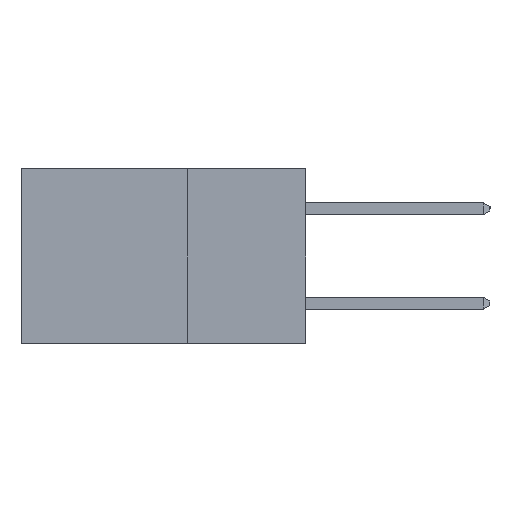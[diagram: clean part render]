
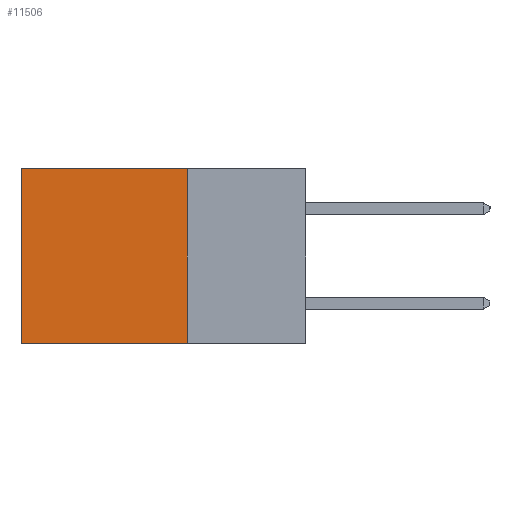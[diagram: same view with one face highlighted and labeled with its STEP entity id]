
A CAD part, left-side view. The second image highlights one B-rep face of the part: STEP entity #11506.
In plain terms, the highlighted planar face has unit normal (-1, 0, 0).
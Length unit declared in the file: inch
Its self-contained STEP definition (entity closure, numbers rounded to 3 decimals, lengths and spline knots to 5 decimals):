
#548 = VECTOR ( 'NONE', #12757, 39.37008 ) ;
#884 = ORIENTED_EDGE ( 'NONE', *, *, #16529, .T. ) ;
#2246 = CARTESIAN_POINT ( 'NONE',  ( 0.2615, 0.25, -0.37 ) ) ;
#3835 = LINE ( 'NONE', #18355, #8710 ) ;
#4700 = DIRECTION ( 'NONE',  ( 1., 0., 0. ) ) ;
#5095 = PLANE ( 'NONE',  #11170 ) ;
#5743 = ORIENTED_EDGE ( 'NONE', *, *, #10610, .F. ) ;
#5829 = LINE ( 'NONE', #16227, #17690 ) ;
#7316 = CARTESIAN_POINT ( 'NONE',  ( 0.2615, 0.6, 0. ) ) ;
#7405 = ORIENTED_EDGE ( 'NONE', *, *, #15174, .T. ) ;
#7695 = DIRECTION ( 'NONE',  ( 0., 1., 0. ) ) ;
#7808 = DIRECTION ( 'NONE',  ( 0., 1., 0. ) ) ;
#8710 = VECTOR ( 'NONE', #9820, 39.37008 ) ;
#8884 = ORIENTED_EDGE ( 'NONE', *, *, #15181, .F. ) ;
#9820 = DIRECTION ( 'NONE',  ( 0., 0., -1. ) ) ;
#10110 = VERTEX_POINT ( 'NONE', #13282 ) ;
#10532 = VERTEX_POINT ( 'NONE', #11553 ) ;
#10610 = EDGE_CURVE ( 'NONE', #14401, #10532, #5829, .T. ) ;
#10849 = LINE ( 'NONE', #15454, #18750 ) ;
#10894 = DIRECTION ( 'NONE',  ( 0., 0., -1. ) ) ;
#11170 = AXIS2_PLACEMENT_3D ( 'NONE', #13619, #4700, #10894 ) ;
#11506 = ADVANCED_FACE ( 'NONE', ( #16667 ), #5095, .F. ) ;
#11553 = CARTESIAN_POINT ( 'NONE',  ( 0.2615, 0.6, -0.37 ) ) ;
#12578 = LINE ( 'NONE', #15428, #548 ) ;
#12757 = DIRECTION ( 'NONE',  ( 0., 0., -1. ) ) ;
#13282 = CARTESIAN_POINT ( 'NONE',  ( 0.2615, 0.25, 0. ) ) ;
#13619 = CARTESIAN_POINT ( 'NONE',  ( 0.2615, 0.25, -0.37 ) ) ;
#13737 = VERTEX_POINT ( 'NONE', #7316 ) ;
#14401 = VERTEX_POINT ( 'NONE', #2246 ) ;
#15174 = EDGE_CURVE ( 'NONE', #13737, #10532, #12578, .T. ) ;
#15181 = EDGE_CURVE ( 'NONE', #10110, #14401, #3835, .T. ) ;
#15428 = CARTESIAN_POINT ( 'NONE',  ( 0.2615, 0.6, -0.37 ) ) ;
#15454 = CARTESIAN_POINT ( 'NONE',  ( 0.2615, 0.25, 0. ) ) ;
#16227 = CARTESIAN_POINT ( 'NONE',  ( 0.2615, 0.25, -0.37 ) ) ;
#16529 = EDGE_CURVE ( 'NONE', #10110, #13737, #10849, .T. ) ;
#16667 = FACE_OUTER_BOUND ( 'NONE', #18345, .T. ) ;
#17690 = VECTOR ( 'NONE', #7695, 39.37008 ) ;
#18345 = EDGE_LOOP ( 'NONE', ( #7405, #5743, #8884, #884 ) ) ;
#18355 = CARTESIAN_POINT ( 'NONE',  ( 0.2615, 0.25, -0.37 ) ) ;
#18750 = VECTOR ( 'NONE', #7808, 39.37008 ) ;
